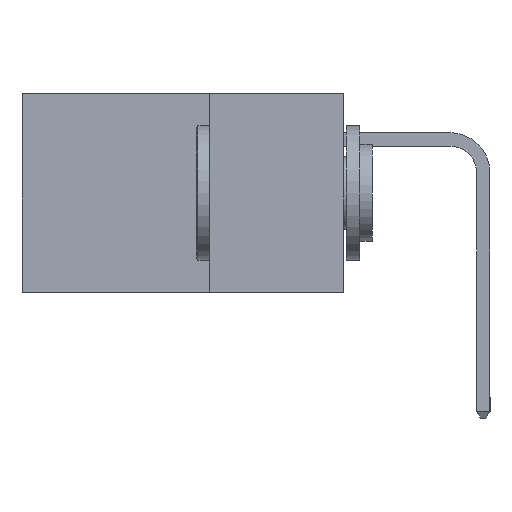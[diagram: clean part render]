
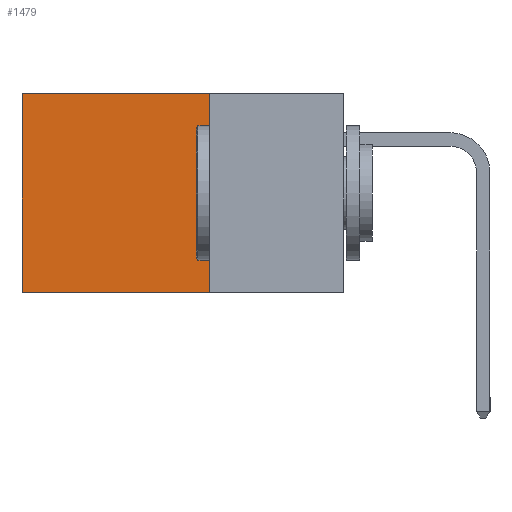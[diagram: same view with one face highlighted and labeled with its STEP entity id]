
A CAD part, left-side view. The second image highlights one B-rep face of the part: STEP entity #1479.
In plain terms, the highlighted planar face has unit normal (-1, 0, 0).
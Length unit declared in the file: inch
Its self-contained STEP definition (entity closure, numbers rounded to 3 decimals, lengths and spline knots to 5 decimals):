
#1479 = ADVANCED_FACE ( 'NONE', ( #2708 ), #2366, .F. ) ;
#1663 = CARTESIAN_POINT ( 'NONE',  ( 0.2615, 0.6, -0.37 ) ) ;
#2194 = DIRECTION ( 'NONE',  ( 0., 0., -1. ) ) ;
#2366 = PLANE ( 'NONE',  #8820 ) ;
#2708 = FACE_OUTER_BOUND ( 'NONE', #17909, .T. ) ;
#3665 = VERTEX_POINT ( 'NONE', #1663 ) ;
#3697 = CARTESIAN_POINT ( 'NONE',  ( 0.2615, 0.25, 0. ) ) ;
#5143 = EDGE_CURVE ( 'NONE', #6632, #9417, #7184, .T. ) ;
#5298 = EDGE_CURVE ( 'NONE', #9417, #3665, #16952, .T. ) ;
#5306 = DIRECTION ( 'NONE',  ( 0., 1., 0. ) ) ;
#5670 = CARTESIAN_POINT ( 'NONE',  ( 0.2615, 0.25, -0.37 ) ) ;
#5703 = DIRECTION ( 'NONE',  ( 0., 0., -1. ) ) ;
#5978 = DIRECTION ( 'NONE',  ( 1., 0., 0. ) ) ;
#6632 = VERTEX_POINT ( 'NONE', #20415 ) ;
#6831 = VERTEX_POINT ( 'NONE', #17535 ) ;
#6883 = VECTOR ( 'NONE', #5306, 39.37008 ) ;
#7184 = LINE ( 'NONE', #13439, #19454 ) ;
#8820 = AXIS2_PLACEMENT_3D ( 'NONE', #13683, #5978, #5703 ) ;
#9417 = VERTEX_POINT ( 'NONE', #15298 ) ;
#9744 = ORIENTED_EDGE ( 'NONE', *, *, #5143, .F. ) ;
#10048 = EDGE_CURVE ( 'NONE', #6831, #3665, #15002, .T. ) ;
#10529 = DIRECTION ( 'NONE',  ( 0., 1., 0. ) ) ;
#10690 = VECTOR ( 'NONE', #11205, 39.37008 ) ;
#11205 = DIRECTION ( 'NONE',  ( 0., 0., -1. ) ) ;
#12756 = VECTOR ( 'NONE', #10529, 39.37008 ) ;
#12851 = EDGE_CURVE ( 'NONE', #6632, #6831, #19643, .T. ) ;
#13439 = CARTESIAN_POINT ( 'NONE',  ( 0.2615, 0.25, -0.37 ) ) ;
#13683 = CARTESIAN_POINT ( 'NONE',  ( 0.2615, 0.25, -0.37 ) ) ;
#13791 = ORIENTED_EDGE ( 'NONE', *, *, #12851, .T. ) ;
#15002 = LINE ( 'NONE', #17499, #10690 ) ;
#15158 = ORIENTED_EDGE ( 'NONE', *, *, #5298, .F. ) ;
#15298 = CARTESIAN_POINT ( 'NONE',  ( 0.2615, 0.25, -0.37 ) ) ;
#16952 = LINE ( 'NONE', #5670, #12756 ) ;
#17099 = ORIENTED_EDGE ( 'NONE', *, *, #10048, .T. ) ;
#17499 = CARTESIAN_POINT ( 'NONE',  ( 0.2615, 0.6, -0.37 ) ) ;
#17535 = CARTESIAN_POINT ( 'NONE',  ( 0.2615, 0.6, 0. ) ) ;
#17909 = EDGE_LOOP ( 'NONE', ( #17099, #15158, #9744, #13791 ) ) ;
#19454 = VECTOR ( 'NONE', #2194, 39.37008 ) ;
#19643 = LINE ( 'NONE', #3697, #6883 ) ;
#20415 = CARTESIAN_POINT ( 'NONE',  ( 0.2615, 0.25, 0. ) ) ;
